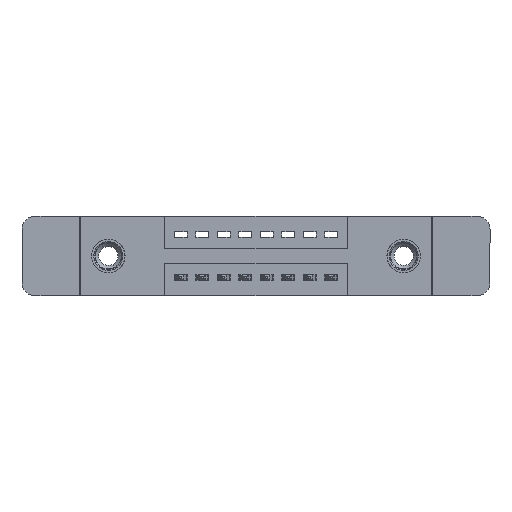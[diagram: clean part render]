
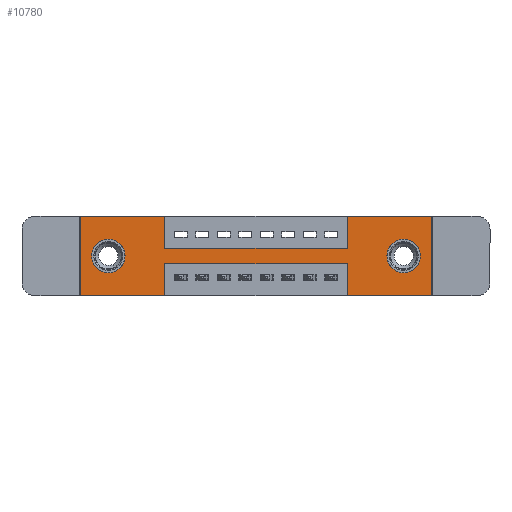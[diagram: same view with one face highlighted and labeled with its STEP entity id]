
A CAD part, front view. The second image highlights one B-rep face of the part: STEP entity #10780.
In plain terms, the highlighted planar face has unit normal (0, -1, 0).
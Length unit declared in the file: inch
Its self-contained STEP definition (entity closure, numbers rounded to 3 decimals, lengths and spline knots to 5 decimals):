
#265 = CARTESIAN_POINT ( 'NONE',  ( 1.635, 0., 0. ) ) ;
#286 = CARTESIAN_POINT ( 'NONE',  ( 0.13, 0., -0.185 ) ) ;
#346 = EDGE_CURVE ( 'NONE', #7439, #9714, #1125, .T. ) ;
#419 = VERTEX_POINT ( 'NONE', #6906 ) ;
#549 = CARTESIAN_POINT ( 'NONE',  ( 1.2425, 0., -0.37 ) ) ;
#576 = DIRECTION ( 'NONE',  ( 0., 0., -1. ) ) ;
#622 = CARTESIAN_POINT ( 'NONE',  ( 1.2425, 0., -0.22 ) ) ;
#731 = VECTOR ( 'NONE', #15812, 39.37008 ) ;
#803 = CARTESIAN_POINT ( 'NONE',  ( 1.635, 0., -0.37 ) ) ;
#880 = VECTOR ( 'NONE', #15081, 39.37008 ) ;
#1067 = VERTEX_POINT ( 'NONE', #803 ) ;
#1125 = LINE ( 'NONE', #3044, #6887 ) ;
#1290 = CARTESIAN_POINT ( 'NONE',  ( 0., 0., -0.37 ) ) ;
#1316 = VERTEX_POINT ( 'NONE', #10301 ) ;
#1436 = ORIENTED_EDGE ( 'NONE', *, *, #4916, .T. ) ;
#1444 = VERTEX_POINT ( 'NONE', #12957 ) ;
#1561 = EDGE_CURVE ( 'NONE', #4443, #1067, #15757, .T. ) ;
#1590 = FACE_BOUND ( 'NONE', #14393, .T. ) ;
#1716 = CARTESIAN_POINT ( 'NONE',  ( 1.505, 0., -0.107 ) ) ;
#1780 = EDGE_CURVE ( 'NONE', #3131, #6128, #11218, .T. ) ;
#1825 = VERTEX_POINT ( 'NONE', #4649 ) ;
#2033 = LINE ( 'NONE', #12763, #6256 ) ;
#2055 = DIRECTION ( 'NONE',  ( 1., 0., 0. ) ) ;
#2121 = ORIENTED_EDGE ( 'NONE', *, *, #3414, .F. ) ;
#2217 = EDGE_CURVE ( 'NONE', #419, #1316, #2624, .T. ) ;
#2375 = LINE ( 'NONE', #12822, #14184 ) ;
#2477 = EDGE_CURVE ( 'NONE', #5130, #1444, #6614, .T. ) ;
#2624 = LINE ( 'NONE', #15025, #880 ) ;
#2820 = DIRECTION ( 'NONE',  ( 0., 1., 0. ) ) ;
#2943 = VERTEX_POINT ( 'NONE', #1716 ) ;
#3044 = CARTESIAN_POINT ( 'NONE',  ( 0.3925, 0., -0.22 ) ) ;
#3131 = VERTEX_POINT ( 'NONE', #7407 ) ;
#3191 = VERTEX_POINT ( 'NONE', #8669 ) ;
#3310 = CARTESIAN_POINT ( 'NONE',  ( 0.3925, 0., -0.15 ) ) ;
#3408 = CARTESIAN_POINT ( 'NONE',  ( 0., 0., -0.37 ) ) ;
#3414 = EDGE_CURVE ( 'NONE', #1316, #4797, #12108, .T. ) ;
#4374 = DIRECTION ( 'NONE',  ( 0., 1., 0. ) ) ;
#4443 = VERTEX_POINT ( 'NONE', #11590 ) ;
#4561 = ORIENTED_EDGE ( 'NONE', *, *, #13547, .F. ) ;
#4646 = DIRECTION ( 'NONE',  ( 0., 1., 0. ) ) ;
#4649 = CARTESIAN_POINT ( 'NONE',  ( 0.3925, 0., -0.15 ) ) ;
#4797 = VERTEX_POINT ( 'NONE', #10990 ) ;
#4831 = FACE_BOUND ( 'NONE', #8820, .T. ) ;
#4916 = EDGE_CURVE ( 'NONE', #2943, #10504, #6523, .T. ) ;
#5130 = VERTEX_POINT ( 'NONE', #6997 ) ;
#5393 = ORIENTED_EDGE ( 'NONE', *, *, #1561, .F. ) ;
#5430 = EDGE_CURVE ( 'NONE', #1067, #6344, #8064, .T. ) ;
#5511 = DIRECTION ( 'NONE',  ( 0., 0., -1. ) ) ;
#5814 = CARTESIAN_POINT ( 'NONE',  ( 1.505, 0., -0.185 ) ) ;
#5973 = ORIENTED_EDGE ( 'NONE', *, *, #14123, .F. ) ;
#5992 = CARTESIAN_POINT ( 'NONE',  ( 0.13, 0., -0.185 ) ) ;
#6128 = VERTEX_POINT ( 'NONE', #9362 ) ;
#6182 = FACE_OUTER_BOUND ( 'NONE', #11241, .T. ) ;
#6256 = VECTOR ( 'NONE', #15139, 39.37008 ) ;
#6344 = VERTEX_POINT ( 'NONE', #549 ) ;
#6494 = EDGE_CURVE ( 'NONE', #1825, #3131, #9342, .T. ) ;
#6523 = CIRCLE ( 'NONE', #8051, 0.078 ) ;
#6606 = ORIENTED_EDGE ( 'NONE', *, *, #2217, .F. ) ;
#6614 = CIRCLE ( 'NONE', #14815, 0.078 ) ;
#6887 = VECTOR ( 'NONE', #15186, 39.37008 ) ;
#6906 = CARTESIAN_POINT ( 'NONE',  ( 0., 0., -0.37 ) ) ;
#6922 = CARTESIAN_POINT ( 'NONE',  ( 1.2425, 0., 0. ) ) ;
#6946 = LINE ( 'NONE', #10618, #10358 ) ;
#6997 = CARTESIAN_POINT ( 'NONE',  ( 0.13, 0., -0.263 ) ) ;
#7038 = VECTOR ( 'NONE', #14780, 39.37008 ) ;
#7095 = ORIENTED_EDGE ( 'NONE', *, *, #11160, .T. ) ;
#7141 = ORIENTED_EDGE ( 'NONE', *, *, #2477, .T. ) ;
#7165 = ORIENTED_EDGE ( 'NONE', *, *, #8516, .F. ) ;
#7308 = CARTESIAN_POINT ( 'NONE',  ( 0.3925, 0., -0.22 ) ) ;
#7407 = CARTESIAN_POINT ( 'NONE',  ( 1.2425, 0., -0.15 ) ) ;
#7439 = VERTEX_POINT ( 'NONE', #622 ) ;
#8051 = AXIS2_PLACEMENT_3D ( 'NONE', #11686, #4374, #576 ) ;
#8064 = LINE ( 'NONE', #12577, #13174 ) ;
#8164 = CARTESIAN_POINT ( 'NONE',  ( 1.2425, 0., -0.37 ) ) ;
#8500 = VECTOR ( 'NONE', #2055, 39.37008 ) ;
#8516 = EDGE_CURVE ( 'NONE', #9714, #3191, #2033, .T. ) ;
#8519 = DIRECTION ( 'NONE',  ( -1., 0., 0. ) ) ;
#8669 = CARTESIAN_POINT ( 'NONE',  ( 0.3925, 0., -0.37 ) ) ;
#8820 = EDGE_LOOP ( 'NONE', ( #1436, #13260 ) ) ;
#9138 = VECTOR ( 'NONE', #9515, 39.37008 ) ;
#9313 = AXIS2_PLACEMENT_3D ( 'NONE', #286, #2820, #13726 ) ;
#9342 = LINE ( 'NONE', #3310, #731 ) ;
#9362 = CARTESIAN_POINT ( 'NONE',  ( 1.2425, 0., 0. ) ) ;
#9380 = DIRECTION ( 'NONE',  ( 0., 0., 1. ) ) ;
#9515 = DIRECTION ( 'NONE',  ( 0., 0., 1. ) ) ;
#9714 = VERTEX_POINT ( 'NONE', #7308 ) ;
#9941 = ORIENTED_EDGE ( 'NONE', *, *, #10815, .F. ) ;
#10301 = CARTESIAN_POINT ( 'NONE',  ( 0., 0., 0. ) ) ;
#10358 = VECTOR ( 'NONE', #11858, 39.37008 ) ;
#10417 = ORIENTED_EDGE ( 'NONE', *, *, #346, .F. ) ;
#10504 = VERTEX_POINT ( 'NONE', #11323 ) ;
#10565 = ORIENTED_EDGE ( 'NONE', *, *, #12217, .F. ) ;
#10618 = CARTESIAN_POINT ( 'NONE',  ( 0., 0., 0. ) ) ;
#10780 = ADVANCED_FACE ( 'NONE', ( #4831, #1590, #6182 ), #15390, .T. ) ;
#10815 = EDGE_CURVE ( 'NONE', #6128, #4443, #6946, .T. ) ;
#10835 = ORIENTED_EDGE ( 'NONE', *, *, #5430, .F. ) ;
#10990 = CARTESIAN_POINT ( 'NONE',  ( 0.3925, 0., 0. ) ) ;
#11160 = EDGE_CURVE ( 'NONE', #1444, #5130, #11702, .T. ) ;
#11218 = LINE ( 'NONE', #6922, #9138 ) ;
#11241 = EDGE_LOOP ( 'NONE', ( #7165, #10417, #4561, #10835, #5393, #9941, #13920, #12945, #5973, #2121, #6606, #10565 ) ) ;
#11323 = CARTESIAN_POINT ( 'NONE',  ( 1.505, 0., -0.263 ) ) ;
#11403 = DIRECTION ( 'NONE',  ( -1., 0., 0. ) ) ;
#11579 = LINE ( 'NONE', #1290, #13824 ) ;
#11590 = CARTESIAN_POINT ( 'NONE',  ( 1.635, 0., 0. ) ) ;
#11686 = CARTESIAN_POINT ( 'NONE',  ( 1.505, 0., -0.185 ) ) ;
#11702 = CIRCLE ( 'NONE', #9313, 0.078 ) ;
#11858 = DIRECTION ( 'NONE',  ( 1., 0., 0. ) ) ;
#11901 = DIRECTION ( 'NONE',  ( 0., 0., -1. ) ) ;
#12093 = CIRCLE ( 'NONE', #15033, 0.078 ) ;
#12108 = LINE ( 'NONE', #14129, #8500 ) ;
#12217 = EDGE_CURVE ( 'NONE', #3191, #419, #11579, .T. ) ;
#12231 = DIRECTION ( 'NONE',  ( 0., 0., 1. ) ) ;
#12332 = LINE ( 'NONE', #8164, #14202 ) ;
#12577 = CARTESIAN_POINT ( 'NONE',  ( 0., 0., -0.37 ) ) ;
#12763 = CARTESIAN_POINT ( 'NONE',  ( 0.3925, 0., -0.37 ) ) ;
#12822 = CARTESIAN_POINT ( 'NONE',  ( 0.3925, 0., 0. ) ) ;
#12945 = ORIENTED_EDGE ( 'NONE', *, *, #6494, .F. ) ;
#12957 = CARTESIAN_POINT ( 'NONE',  ( 0.13, 0., -0.107 ) ) ;
#13174 = VECTOR ( 'NONE', #11403, 39.37008 ) ;
#13260 = ORIENTED_EDGE ( 'NONE', *, *, #14345, .T. ) ;
#13373 = DIRECTION ( 'NONE',  ( 0., 1., 0. ) ) ;
#13547 = EDGE_CURVE ( 'NONE', #6344, #7439, #12332, .T. ) ;
#13726 = DIRECTION ( 'NONE',  ( 0., 0., 1. ) ) ;
#13750 = AXIS2_PLACEMENT_3D ( 'NONE', #3408, #15344, #11901 ) ;
#13824 = VECTOR ( 'NONE', #8519, 39.37008 ) ;
#13920 = ORIENTED_EDGE ( 'NONE', *, *, #1780, .F. ) ;
#14123 = EDGE_CURVE ( 'NONE', #4797, #1825, #2375, .T. ) ;
#14129 = CARTESIAN_POINT ( 'NONE',  ( 0., 0., 0. ) ) ;
#14184 = VECTOR ( 'NONE', #5511, 39.37008 ) ;
#14202 = VECTOR ( 'NONE', #9380, 39.37008 ) ;
#14345 = EDGE_CURVE ( 'NONE', #10504, #2943, #12093, .T. ) ;
#14393 = EDGE_LOOP ( 'NONE', ( #7095, #7141 ) ) ;
#14780 = DIRECTION ( 'NONE',  ( 0., 0., -1. ) ) ;
#14815 = AXIS2_PLACEMENT_3D ( 'NONE', #5992, #13373, #12231 ) ;
#15025 = CARTESIAN_POINT ( 'NONE',  ( 0., 0., 0. ) ) ;
#15033 = AXIS2_PLACEMENT_3D ( 'NONE', #5814, #4646, #15605 ) ;
#15081 = DIRECTION ( 'NONE',  ( 0., 0., 1. ) ) ;
#15139 = DIRECTION ( 'NONE',  ( 0., 0., -1. ) ) ;
#15186 = DIRECTION ( 'NONE',  ( -1., 0., 0. ) ) ;
#15344 = DIRECTION ( 'NONE',  ( 0., -1., 0. ) ) ;
#15390 = PLANE ( 'NONE',  #13750 ) ;
#15605 = DIRECTION ( 'NONE',  ( 0., 0., -1. ) ) ;
#15757 = LINE ( 'NONE', #265, #7038 ) ;
#15812 = DIRECTION ( 'NONE',  ( 1., 0., 0. ) ) ;
